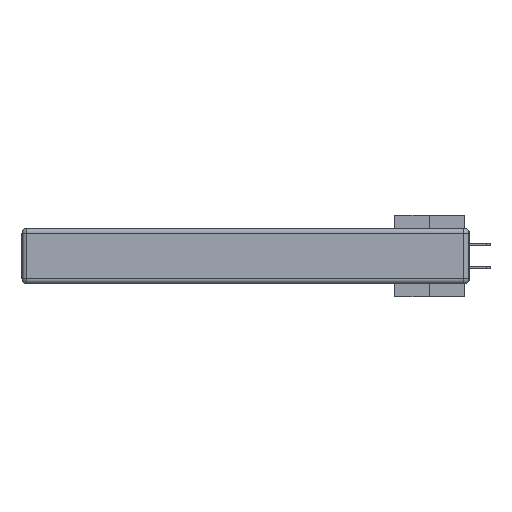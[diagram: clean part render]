
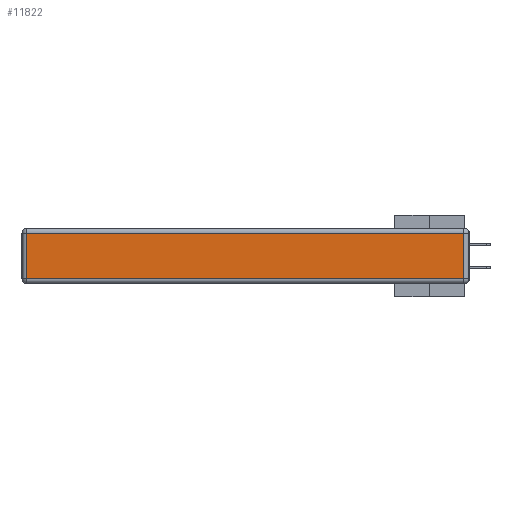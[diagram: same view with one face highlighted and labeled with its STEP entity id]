
A CAD part, left-side view. The second image highlights one B-rep face of the part: STEP entity #11822.
In plain terms, the highlighted planar face has unit normal (-1, 0, 0).
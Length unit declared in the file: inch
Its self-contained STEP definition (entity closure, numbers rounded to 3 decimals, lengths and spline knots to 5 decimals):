
#116 = VECTOR ( 'NONE', #32624, 39.37008 ) ;
#1613 = CARTESIAN_POINT ( 'NONE',  ( 0., 0., -0.313 ) ) ;
#2837 = EDGE_CURVE ( 'NONE', #8027, #9195, #28408, .T. ) ;
#4138 = ORIENTED_EDGE ( 'NONE', *, *, #2837, .T. ) ;
#5643 = CARTESIAN_POINT ( 'NONE',  ( 0., 0., -0.343 ) ) ;
#5677 = LINE ( 'NONE', #26408, #31422 ) ;
#6843 = EDGE_LOOP ( 'NONE', ( #33327, #10529, #4138, #33130 ) ) ;
#7462 = LINE ( 'NONE', #13355, #116 ) ;
#7665 = VERTEX_POINT ( 'NONE', #32629 ) ;
#7700 = CARTESIAN_POINT ( 'NONE',  ( 0., 2.72, -0.03 ) ) ;
#8027 = VERTEX_POINT ( 'NONE', #24280 ) ;
#8891 = DIRECTION ( 'NONE',  ( 0., 1., 0. ) ) ;
#9195 = VERTEX_POINT ( 'NONE', #7700 ) ;
#10529 = ORIENTED_EDGE ( 'NONE', *, *, #32761, .T. ) ;
#10725 = VECTOR ( 'NONE', #8891, 39.37008 ) ;
#11822 = ADVANCED_FACE ( 'NONE', ( #26096 ), #22037, .T. ) ;
#12421 = EDGE_CURVE ( 'NONE', #18594, #7665, #23474, .T. ) ;
#13355 = CARTESIAN_POINT ( 'NONE',  ( 0., 2.72, -0.343 ) ) ;
#18294 = EDGE_CURVE ( 'NONE', #9195, #18594, #7462, .T. ) ;
#18594 = VERTEX_POINT ( 'NONE', #29128 ) ;
#21176 = DIRECTION ( 'NONE',  ( 0., -1., 0. ) ) ;
#22037 = PLANE ( 'NONE',  #23797 ) ;
#23474 = LINE ( 'NONE', #1613, #35541 ) ;
#23797 = AXIS2_PLACEMENT_3D ( 'NONE', #5643, #26153, #26847 ) ;
#24280 = CARTESIAN_POINT ( 'NONE',  ( 0., 0.03, -0.03 ) ) ;
#26096 = FACE_OUTER_BOUND ( 'NONE', #6843, .T. ) ;
#26153 = DIRECTION ( 'NONE',  ( -1., 0., 0. ) ) ;
#26408 = CARTESIAN_POINT ( 'NONE',  ( 0., 0.03, -0.343 ) ) ;
#26847 = DIRECTION ( 'NONE',  ( 0., 0., 1. ) ) ;
#28205 = CARTESIAN_POINT ( 'NONE',  ( 0., 2.75, -0.03 ) ) ;
#28408 = LINE ( 'NONE', #28205, #10725 ) ;
#29128 = CARTESIAN_POINT ( 'NONE',  ( 0., 2.72, -0.313 ) ) ;
#31422 = VECTOR ( 'NONE', #34965, 39.37008 ) ;
#32624 = DIRECTION ( 'NONE',  ( 0., 0., -1. ) ) ;
#32629 = CARTESIAN_POINT ( 'NONE',  ( 0., 0.03, -0.313 ) ) ;
#32761 = EDGE_CURVE ( 'NONE', #7665, #8027, #5677, .T. ) ;
#33130 = ORIENTED_EDGE ( 'NONE', *, *, #18294, .T. ) ;
#33327 = ORIENTED_EDGE ( 'NONE', *, *, #12421, .T. ) ;
#34965 = DIRECTION ( 'NONE',  ( 0., 0., 1. ) ) ;
#35541 = VECTOR ( 'NONE', #21176, 39.37008 ) ;
